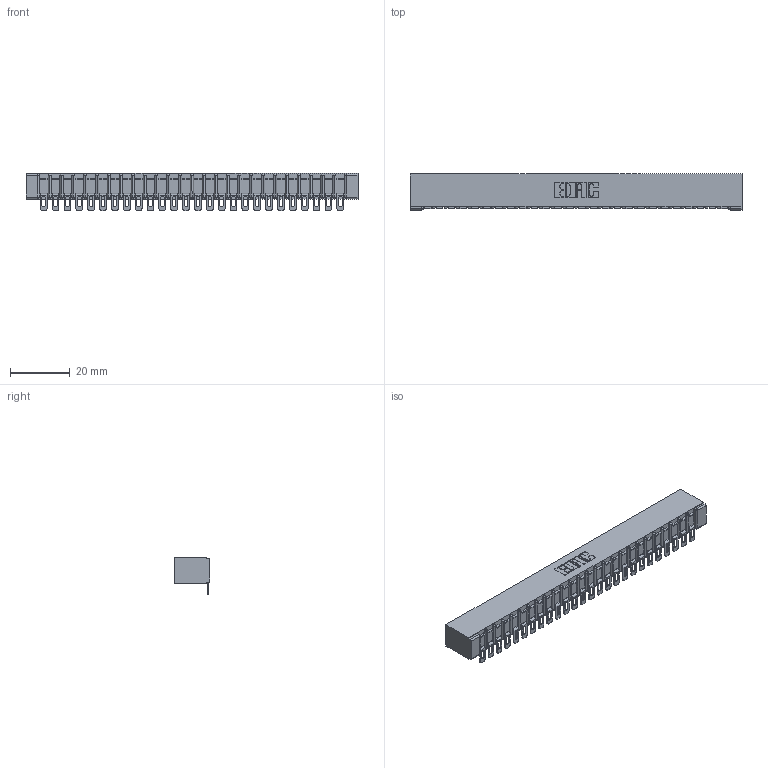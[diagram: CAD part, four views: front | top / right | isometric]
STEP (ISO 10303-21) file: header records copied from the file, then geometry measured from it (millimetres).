
FILE_DESCRIPTION (( 'STEP AP203' ), '1' );
FILE_NAME ('307-026-554-101.STEP', '2018-08-04T14:06:21', ( '' ), ( '' ), 'SwSTEP 2.0', 'SolidWorks 2016', '' );
FILE_SCHEMA (( 'CONFIG_CONTROL_DESIGN' ));
Length unit declared in the file: inch
Products named in the file (3): 307 Part_No Mounting Lugs; 307-290-002_554; 307-026-554-101
Assembly tree (27 placements, depth 2):
  307-026-554-101
    307 Part_No Mounting Lugs
    307-290-002_554  x26
Bounding box: 110.9 x 12.01 x 12.52 mm (x, y, z)
Volume: 7574.9 mm3; surface area: 14614.1 mm2
Topology: 27 solids, 27 shells, 2243 faces, 6877 edges, 4510 vertices
Faces by surface type: plane 1262, cylinder 927, sphere 54
Entity records: 24949 total; most frequent: CARTESIAN_POINT 4206, ORIENTED_EDGE 4196, DIRECTION 4098, EDGE_CURVE 2098, VECTOR 1594, LINE 1594, VERTEX_POINT 1360, AXIS2_PLACEMENT_3D 1252
